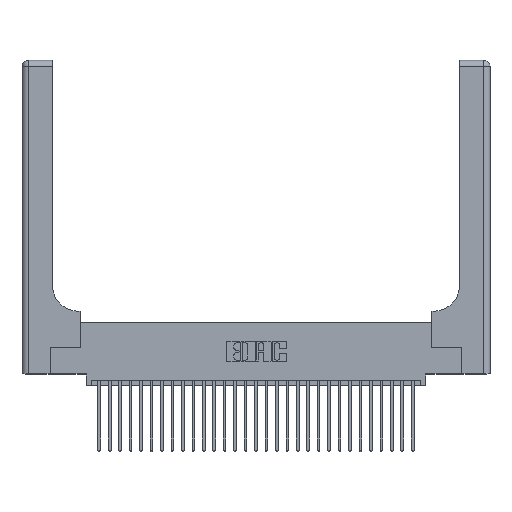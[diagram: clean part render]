
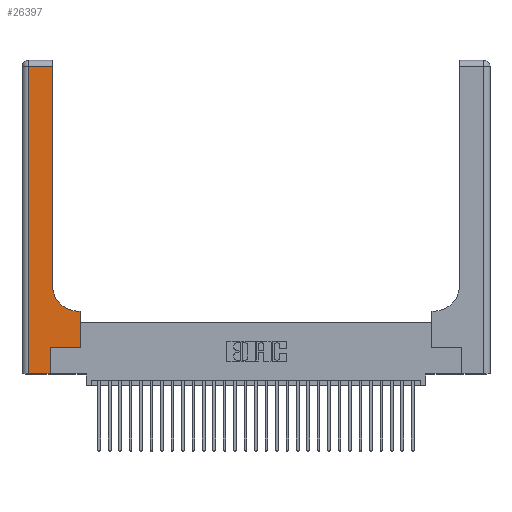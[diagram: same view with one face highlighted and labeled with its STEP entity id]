
A CAD part, top view. The second image highlights one B-rep face of the part: STEP entity #26397.
In plain terms, the highlighted planar face has unit normal (0, 0, 1).
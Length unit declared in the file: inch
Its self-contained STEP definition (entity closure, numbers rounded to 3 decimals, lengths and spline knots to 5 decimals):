
#382 = AXIS2_PLACEMENT_3D ( 'NONE', #28776, #28467, #18840 ) ;
#775 = VECTOR ( 'NONE', #8673, 39.37008 ) ;
#941 = CARTESIAN_POINT ( 'NONE',  ( 0.2915, 2.94, 0.37 ) ) ;
#1190 = CARTESIAN_POINT ( 'NONE',  ( 0.5585, 0.6, 0.37 ) ) ;
#1624 = CARTESIAN_POINT ( 'NONE',  ( 0.5585, 0.25, 0.37 ) ) ;
#2042 = DIRECTION ( 'NONE',  ( 0., 1., 0. ) ) ;
#2790 = VERTEX_POINT ( 'NONE', #4832 ) ;
#3942 = EDGE_CURVE ( 'NONE', #20363, #5303, #21095, .T. ) ;
#4057 = CARTESIAN_POINT ( 'NONE',  ( 0.06, 2.94, 0.37 ) ) ;
#4281 = VECTOR ( 'NONE', #23309, 39.37008 ) ;
#4413 = CARTESIAN_POINT ( 'NONE',  ( 0.2915, 3., 0.37 ) ) ;
#4469 = ORIENTED_EDGE ( 'NONE', *, *, #14275, .T. ) ;
#4832 = CARTESIAN_POINT ( 'NONE',  ( 0.2915, 0.85, 0.37 ) ) ;
#5034 = CARTESIAN_POINT ( 'NONE',  ( 0.06, 3., 0.37 ) ) ;
#5182 = CARTESIAN_POINT ( 'NONE',  ( 0., 0., 0.37 ) ) ;
#5263 = LINE ( 'NONE', #4413, #9064 ) ;
#5303 = VERTEX_POINT ( 'NONE', #8776 ) ;
#5597 = DIRECTION ( 'NONE',  ( 1., 0., 0. ) ) ;
#5635 = ORIENTED_EDGE ( 'NONE', *, *, #16341, .T. ) ;
#6130 = EDGE_LOOP ( 'NONE', ( #8676, #5635, #20860, #11509, #20720, #4469, #10680, #11818, #14430 ) ) ;
#6588 = CARTESIAN_POINT ( 'NONE',  ( 0., 3., 0.37 ) ) ;
#7458 = VERTEX_POINT ( 'NONE', #941 ) ;
#8673 = DIRECTION ( 'NONE',  ( -1., 0., 0. ) ) ;
#8676 = ORIENTED_EDGE ( 'NONE', *, *, #30814, .T. ) ;
#8776 = CARTESIAN_POINT ( 'NONE',  ( 0.269, 0., 0.37 ) ) ;
#9064 = VECTOR ( 'NONE', #2042, 39.37008 ) ;
#9293 = AXIS2_PLACEMENT_3D ( 'NONE', #6588, #30340, #13771 ) ;
#9369 = CARTESIAN_POINT ( 'NONE',  ( 0.06, 0., 0.37 ) ) ;
#9530 = VECTOR ( 'NONE', #15119, 39.37008 ) ;
#10680 = ORIENTED_EDGE ( 'NONE', *, *, #28275, .T. ) ;
#10681 = CARTESIAN_POINT ( 'NONE',  ( 0.5585, 0.25, 0.37 ) ) ;
#11509 = ORIENTED_EDGE ( 'NONE', *, *, #3942, .T. ) ;
#11818 = ORIENTED_EDGE ( 'NONE', *, *, #22946, .T. ) ;
#12322 = VERTEX_POINT ( 'NONE', #1190 ) ;
#12990 = VERTEX_POINT ( 'NONE', #10681 ) ;
#13451 = FACE_OUTER_BOUND ( 'NONE', #6130, .T. ) ;
#13456 = CARTESIAN_POINT ( 'NONE',  ( 0.5415, 0.6, 0.37 ) ) ;
#13692 = VECTOR ( 'NONE', #18506, 39.37008 ) ;
#13771 = DIRECTION ( 'NONE',  ( -1., 0., 0. ) ) ;
#14017 = VECTOR ( 'NONE', #19146, 39.37008 ) ;
#14275 = EDGE_CURVE ( 'NONE', #27611, #12990, #29835, .T. ) ;
#14430 = ORIENTED_EDGE ( 'NONE', *, *, #14523, .T. ) ;
#14523 = EDGE_CURVE ( 'NONE', #24229, #2790, #19295, .T. ) ;
#14803 = LINE ( 'NONE', #1624, #13692 ) ;
#14909 = CARTESIAN_POINT ( 'NONE',  ( 0., 2.94, 0.37 ) ) ;
#15119 = DIRECTION ( 'NONE',  ( 0., 1., 0. ) ) ;
#15137 = LINE ( 'NONE', #27430, #775 ) ;
#16262 = VECTOR ( 'NONE', #5597, 39.37008 ) ;
#16341 = EDGE_CURVE ( 'NONE', #7458, #26905, #29684, .T. ) ;
#18506 = DIRECTION ( 'NONE',  ( 0., 1., 0. ) ) ;
#18840 = DIRECTION ( 'NONE',  ( 1., 0., 0. ) ) ;
#19146 = DIRECTION ( 'NONE',  ( 0., -1., 0. ) ) ;
#19295 = CIRCLE ( 'NONE', #382, 0.25 ) ;
#20142 = CARTESIAN_POINT ( 'NONE',  ( 0.269, 0., 0.37 ) ) ;
#20363 = VERTEX_POINT ( 'NONE', #9369 ) ;
#20416 = LINE ( 'NONE', #20142, #9530 ) ;
#20720 = ORIENTED_EDGE ( 'NONE', *, *, #22083, .T. ) ;
#20860 = ORIENTED_EDGE ( 'NONE', *, *, #29426, .T. ) ;
#21095 = LINE ( 'NONE', #5182, #16262 ) ;
#22083 = EDGE_CURVE ( 'NONE', #5303, #27611, #20416, .T. ) ;
#22564 = PLANE ( 'NONE',  #9293 ) ;
#22946 = EDGE_CURVE ( 'NONE', #12322, #24229, #15137, .T. ) ;
#23309 = DIRECTION ( 'NONE',  ( 1., 0., 0. ) ) ;
#23346 = CARTESIAN_POINT ( 'NONE',  ( 0.269, 0.25, 0.37 ) ) ;
#23693 = VECTOR ( 'NONE', #24629, 39.37008 ) ;
#24229 = VERTEX_POINT ( 'NONE', #13456 ) ;
#24629 = DIRECTION ( 'NONE',  ( -1., 0., 0. ) ) ;
#25906 = CARTESIAN_POINT ( 'NONE',  ( 0.269, 0.25, 0.37 ) ) ;
#26397 = ADVANCED_FACE ( 'NONE', ( #13451 ), #22564, .F. ) ;
#26905 = VERTEX_POINT ( 'NONE', #4057 ) ;
#27430 = CARTESIAN_POINT ( 'NONE',  ( 0.2915, 0.6, 0.37 ) ) ;
#27611 = VERTEX_POINT ( 'NONE', #23346 ) ;
#28275 = EDGE_CURVE ( 'NONE', #12990, #12322, #14803, .T. ) ;
#28467 = DIRECTION ( 'NONE',  ( 0., 0., -1. ) ) ;
#28672 = LINE ( 'NONE', #5034, #14017 ) ;
#28776 = CARTESIAN_POINT ( 'NONE',  ( 0.5415, 0.85, 0.37 ) ) ;
#29426 = EDGE_CURVE ( 'NONE', #26905, #20363, #28672, .T. ) ;
#29684 = LINE ( 'NONE', #14909, #23693 ) ;
#29835 = LINE ( 'NONE', #25906, #4281 ) ;
#30340 = DIRECTION ( 'NONE',  ( 0., 0., -1. ) ) ;
#30814 = EDGE_CURVE ( 'NONE', #2790, #7458, #5263, .T. ) ;
